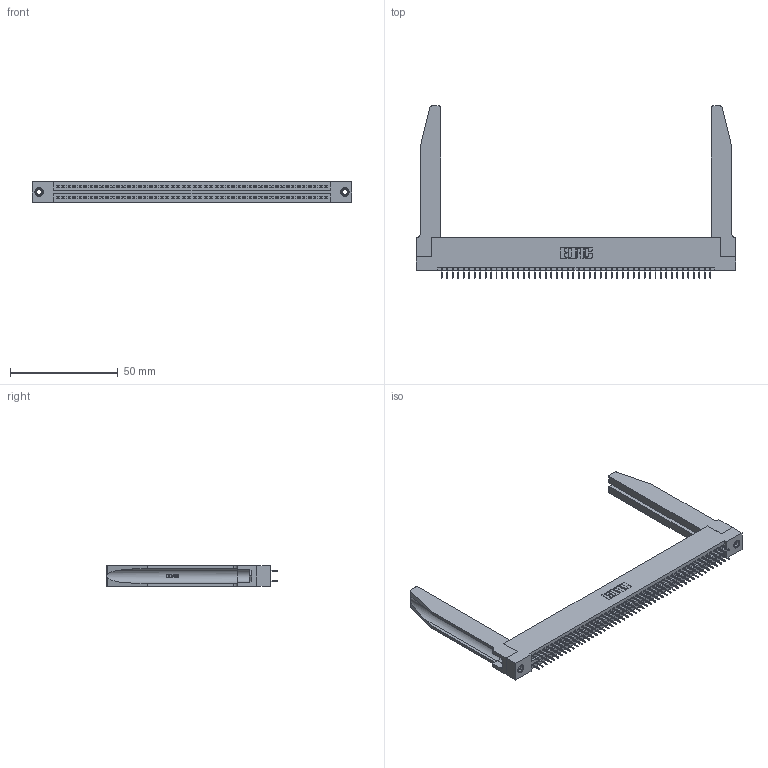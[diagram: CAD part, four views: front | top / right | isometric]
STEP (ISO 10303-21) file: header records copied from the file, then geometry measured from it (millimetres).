
FILE_DESCRIPTION (( 'STEP AP203' ), '1' );
FILE_NAME ('395-100-525-278.STEP', '2020-09-25T16:10:43', ( '' ), ( '' ), 'SwSTEP 2.0', 'SolidWorks 2020', '' );
FILE_SCHEMA (( 'CONFIG_CONTROL_DESIGN' ));
Length unit declared in the file: inch
Products named in the file (5): 345 Part_Flush Mounting Lugs - 0.156 Dia-TH; 345-250-001_345-250-001-102; 395-100-525-278; 345-292-001_345-293-125; 345-220-078_345-220-078
Assembly tree (105 placements, depth 2):
  395-100-525-278
    345 Part_Flush Mounting Lugs - 0.156 Dia-TH
    345-292-001_345-293-125  x100
    345-250-001_345-250-001-102  x2
    345-220-078_345-220-078  x2
Bounding box: 148.23 x 79.68 x 9.4 mm (x, y, z)
Volume: 22079.7 mm3; surface area: 27648.9 mm2
Topology: 105 solids, 105 shells, 5760 faces, 16249 edges, 10422 vertices
Faces by surface type: plane 4122, cylinder 1586, bspline 36, cone 12, torus 4
Entity records: 42968 total; most frequent: CARTESIAN_POINT 8111, ORIENTED_EDGE 6942, DIRECTION 6137, EDGE_CURVE 3471, VECTOR 3049, LINE 3049, VERTEX_POINT 2304, AXIS2_PLACEMENT_3D 1544
